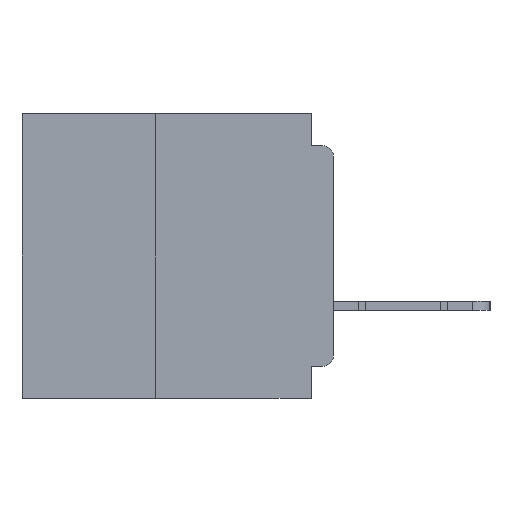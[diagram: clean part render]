
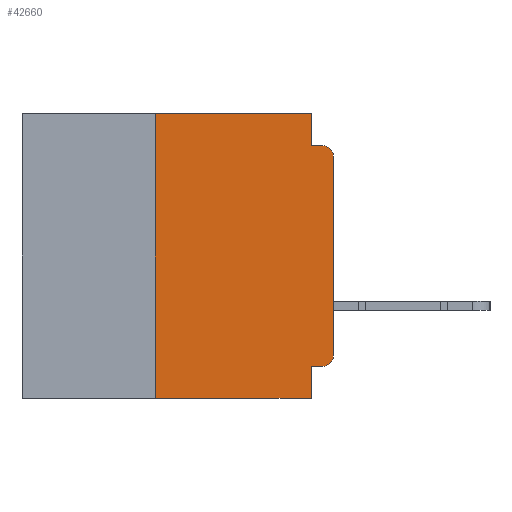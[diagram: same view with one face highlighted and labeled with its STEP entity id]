
A CAD part, left-side view. The second image highlights one B-rep face of the part: STEP entity #42660.
In plain terms, the highlighted planar face has unit normal (-1, 0, 0).
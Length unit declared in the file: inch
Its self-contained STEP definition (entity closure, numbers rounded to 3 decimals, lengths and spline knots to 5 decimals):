
#379 = EDGE_CURVE ( 'NONE', #41651, #27319, #54694, .T. ) ;
#446 = ORIENTED_EDGE ( 'NONE', *, *, #379, .F. ) ;
#2101 = EDGE_CURVE ( 'NONE', #2314, #25372, #19366, .T. ) ;
#2314 = VERTEX_POINT ( 'NONE', #41840 ) ;
#2568 = ORIENTED_EDGE ( 'NONE', *, *, #23776, .F. ) ;
#3089 = DIRECTION ( 'NONE',  ( 0., 0., -1. ) ) ;
#3420 = CARTESIAN_POINT ( 'NONE',  ( 0., 0.25, -0.4 ) ) ;
#4557 = VECTOR ( 'NONE', #20262, 39.37008 ) ;
#4840 = CARTESIAN_POINT ( 'NONE',  ( 0., 0.25, -0.4 ) ) ;
#4951 = CARTESIAN_POINT ( 'NONE',  ( 0., 0.437, 0. ) ) ;
#5278 = DIRECTION ( 'NONE',  ( 0., 0., 1. ) ) ;
#5645 = LINE ( 'NONE', #43390, #18185 ) ;
#6692 = LINE ( 'NONE', #32931, #47321 ) ;
#7436 = VERTEX_POINT ( 'NONE', #26071 ) ;
#7770 = CARTESIAN_POINT ( 'NONE',  ( 0., 0., -0.045 ) ) ;
#9514 = CARTESIAN_POINT ( 'NONE',  ( 0., 0., -0.34 ) ) ;
#10224 = EDGE_CURVE ( 'NONE', #26693, #38067, #23469, .T. ) ;
#10947 = CARTESIAN_POINT ( 'NONE',  ( 0., 0.015, -0.045 ) ) ;
#13560 = ORIENTED_EDGE ( 'NONE', *, *, #17744, .T. ) ;
#13785 = ORIENTED_EDGE ( 'NONE', *, *, #10224, .T. ) ;
#16909 = ORIENTED_EDGE ( 'NONE', *, *, #53200, .T. ) ;
#17102 = CARTESIAN_POINT ( 'NONE',  ( 0., 0.437, 0. ) ) ;
#17658 = EDGE_LOOP ( 'NONE', ( #16909, #13785, #53087, #60608, #49188, #446, #13560, #2568, #56632, #63300 ) ) ;
#17744 = EDGE_CURVE ( 'NONE', #41651, #57752, #5645, .T. ) ;
#18185 = VECTOR ( 'NONE', #48677, 39.37008 ) ;
#19366 = CIRCLE ( 'NONE', #41245, 0.015 ) ;
#20237 = VERTEX_POINT ( 'NONE', #44004 ) ;
#20262 = DIRECTION ( 'NONE',  ( 0., 0., 1. ) ) ;
#20539 = CARTESIAN_POINT ( 'NONE',  ( 0., 0.031, -0.4 ) ) ;
#21526 = EDGE_CURVE ( 'NONE', #27319, #56295, #39347, .T. ) ;
#23469 = CIRCLE ( 'NONE', #43158, 0.015 ) ;
#23776 = EDGE_CURVE ( 'NONE', #20237, #57752, #6692, .T. ) ;
#23847 = DIRECTION ( 'NONE',  ( 0., -1., 0. ) ) ;
#25186 = VECTOR ( 'NONE', #51425, 39.37008 ) ;
#25372 = VERTEX_POINT ( 'NONE', #9514 ) ;
#26071 = CARTESIAN_POINT ( 'NONE',  ( 0., 0.031, -0.045 ) ) ;
#26693 = VERTEX_POINT ( 'NONE', #65280 ) ;
#26819 = VECTOR ( 'NONE', #5278, 39.37008 ) ;
#27319 = VERTEX_POINT ( 'NONE', #28531 ) ;
#27411 = DIRECTION ( 'NONE',  ( 0., 0., -1. ) ) ;
#27794 = DIRECTION ( 'NONE',  ( 1., 0., 0. ) ) ;
#28531 = CARTESIAN_POINT ( 'NONE',  ( 0., 0.25, 0. ) ) ;
#29135 = DIRECTION ( 'NONE',  ( 0., 1., 0. ) ) ;
#30149 = AXIS2_PLACEMENT_3D ( 'NONE', #17102, #27794, #64470 ) ;
#31082 = CARTESIAN_POINT ( 'NONE',  ( 0., 0.015, -0.06 ) ) ;
#31352 = CARTESIAN_POINT ( 'NONE',  ( 0., 0.031, 0. ) ) ;
#31456 = FACE_OUTER_BOUND ( 'NONE', #17658, .T. ) ;
#32859 = PLANE ( 'NONE',  #30149 ) ;
#32931 = CARTESIAN_POINT ( 'NONE',  ( 0., 0.031, -0.4 ) ) ;
#34967 = DIRECTION ( 'NONE',  ( -1., 0., 0. ) ) ;
#36383 = DIRECTION ( 'NONE',  ( 0., 0., -1. ) ) ;
#38067 = VERTEX_POINT ( 'NONE', #10947 ) ;
#39347 = LINE ( 'NONE', #4951, #53218 ) ;
#39537 = CARTESIAN_POINT ( 'NONE',  ( 0., 0., -0.355 ) ) ;
#40863 = LINE ( 'NONE', #56601, #25186 ) ;
#41245 = AXIS2_PLACEMENT_3D ( 'NONE', #66317, #34967, #3089 ) ;
#41651 = VERTEX_POINT ( 'NONE', #3420 ) ;
#41840 = CARTESIAN_POINT ( 'NONE',  ( 0., 0.015, -0.355 ) ) ;
#42660 = ADVANCED_FACE ( 'NONE', ( #31456 ), #32859, .F. ) ;
#43158 = AXIS2_PLACEMENT_3D ( 'NONE', #31082, #67732, #36383 ) ;
#43390 = CARTESIAN_POINT ( 'NONE',  ( 0., 0.437, -0.4 ) ) ;
#44004 = CARTESIAN_POINT ( 'NONE',  ( 0., 0.031, -0.355 ) ) ;
#45198 = LINE ( 'NONE', #56974, #4557 ) ;
#47321 = VECTOR ( 'NONE', #27411, 39.37008 ) ;
#48677 = DIRECTION ( 'NONE',  ( 0., -1., 0. ) ) ;
#49188 = ORIENTED_EDGE ( 'NONE', *, *, #21526, .F. ) ;
#50075 = VECTOR ( 'NONE', #29135, 39.37008 ) ;
#50692 = VECTOR ( 'NONE', #23847, 39.37008 ) ;
#51425 = DIRECTION ( 'NONE',  ( 0., 0., -1. ) ) ;
#52329 = LINE ( 'NONE', #7770, #50692 ) ;
#53087 = ORIENTED_EDGE ( 'NONE', *, *, #62791, .F. ) ;
#53200 = EDGE_CURVE ( 'NONE', #25372, #26693, #45198, .T. ) ;
#53218 = VECTOR ( 'NONE', #62620, 39.37008 ) ;
#54694 = LINE ( 'NONE', #4840, #26819 ) ;
#56295 = VERTEX_POINT ( 'NONE', #31352 ) ;
#56601 = CARTESIAN_POINT ( 'NONE',  ( 0., 0.031, 0. ) ) ;
#56632 = ORIENTED_EDGE ( 'NONE', *, *, #57547, .F. ) ;
#56974 = CARTESIAN_POINT ( 'NONE',  ( 0., 0., 0. ) ) ;
#57547 = EDGE_CURVE ( 'NONE', #2314, #20237, #63975, .T. ) ;
#57752 = VERTEX_POINT ( 'NONE', #20539 ) ;
#60608 = ORIENTED_EDGE ( 'NONE', *, *, #62973, .F. ) ;
#62620 = DIRECTION ( 'NONE',  ( 0., -1., 0. ) ) ;
#62791 = EDGE_CURVE ( 'NONE', #7436, #38067, #52329, .T. ) ;
#62973 = EDGE_CURVE ( 'NONE', #56295, #7436, #40863, .T. ) ;
#63300 = ORIENTED_EDGE ( 'NONE', *, *, #2101, .T. ) ;
#63975 = LINE ( 'NONE', #39537, #50075 ) ;
#64470 = DIRECTION ( 'NONE',  ( 0., 0., -1. ) ) ;
#65280 = CARTESIAN_POINT ( 'NONE',  ( 0., 0., -0.06 ) ) ;
#66317 = CARTESIAN_POINT ( 'NONE',  ( 0., 0.015, -0.34 ) ) ;
#67732 = DIRECTION ( 'NONE',  ( -1., 0., 0. ) ) ;
